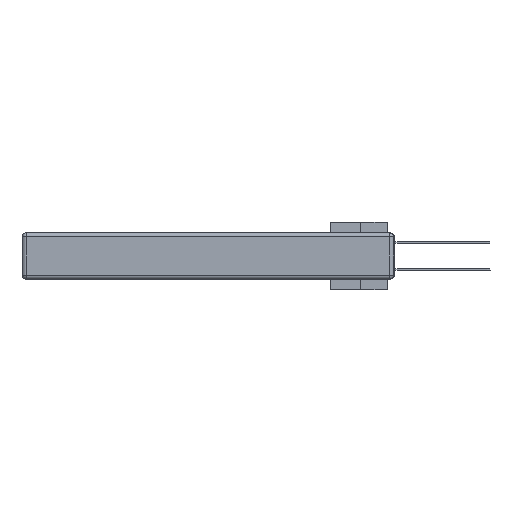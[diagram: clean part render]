
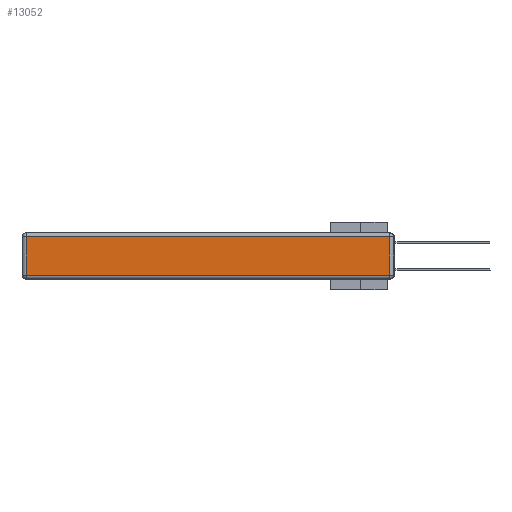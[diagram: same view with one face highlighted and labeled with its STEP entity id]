
A CAD part, left-side view. The second image highlights one B-rep face of the part: STEP entity #13052.
In plain terms, the highlighted planar face has unit normal (-1, 0, 0).
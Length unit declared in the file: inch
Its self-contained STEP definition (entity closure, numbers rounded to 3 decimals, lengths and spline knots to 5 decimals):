
#745 = ORIENTED_EDGE ( 'NONE', *, *, #20664, .T. ) ;
#1275 = DIRECTION ( 'NONE',  ( 0., 0., 1. ) ) ;
#3796 = VERTEX_POINT ( 'NONE', #12516 ) ;
#4359 = LINE ( 'NONE', #39683, #7560 ) ;
#4590 = AXIS2_PLACEMENT_3D ( 'NONE', #29711, #14274, #1275 ) ;
#4713 = PLANE ( 'NONE',  #4590 ) ;
#5811 = ORIENTED_EDGE ( 'NONE', *, *, #21199, .T. ) ;
#6497 = CARTESIAN_POINT ( 'NONE',  ( 0., 2.72, -0.03 ) ) ;
#7235 = VECTOR ( 'NONE', #10796, 39.37008 ) ;
#7301 = ORIENTED_EDGE ( 'NONE', *, *, #15232, .T. ) ;
#7560 = VECTOR ( 'NONE', #21020, 39.37008 ) ;
#10796 = DIRECTION ( 'NONE',  ( 0., 1., 0. ) ) ;
#12516 = CARTESIAN_POINT ( 'NONE',  ( 0., 0.03, -0.03 ) ) ;
#12968 = VERTEX_POINT ( 'NONE', #16524 ) ;
#13052 = ADVANCED_FACE ( 'NONE', ( #35187 ), #4713, .T. ) ;
#13236 = ORIENTED_EDGE ( 'NONE', *, *, #34912, .T. ) ;
#14274 = DIRECTION ( 'NONE',  ( -1., 0., 0. ) ) ;
#15232 = EDGE_CURVE ( 'NONE', #38771, #3796, #17478, .T. ) ;
#16524 = CARTESIAN_POINT ( 'NONE',  ( 0., 2.72, -0.313 ) ) ;
#17478 = LINE ( 'NONE', #39194, #26094 ) ;
#19481 = VERTEX_POINT ( 'NONE', #6497 ) ;
#20664 = EDGE_CURVE ( 'NONE', #12968, #38771, #4359, .T. ) ;
#21020 = DIRECTION ( 'NONE',  ( 0., -1., 0. ) ) ;
#21121 = DIRECTION ( 'NONE',  ( 0., 0., 1. ) ) ;
#21199 = EDGE_CURVE ( 'NONE', #19481, #12968, #36755, .T. ) ;
#24370 = CARTESIAN_POINT ( 'NONE',  ( 0., 0.03, -0.313 ) ) ;
#24452 = VECTOR ( 'NONE', #39593, 39.37008 ) ;
#26094 = VECTOR ( 'NONE', #21121, 39.37008 ) ;
#27986 = CARTESIAN_POINT ( 'NONE',  ( 0., 2.72, -0.343 ) ) ;
#29711 = CARTESIAN_POINT ( 'NONE',  ( 0., 0., -0.343 ) ) ;
#32322 = LINE ( 'NONE', #38404, #7235 ) ;
#32514 = EDGE_LOOP ( 'NONE', ( #745, #7301, #13236, #5811 ) ) ;
#34912 = EDGE_CURVE ( 'NONE', #3796, #19481, #32322, .T. ) ;
#35187 = FACE_OUTER_BOUND ( 'NONE', #32514, .T. ) ;
#36755 = LINE ( 'NONE', #27986, #24452 ) ;
#38404 = CARTESIAN_POINT ( 'NONE',  ( 0., 2.75, -0.03 ) ) ;
#38771 = VERTEX_POINT ( 'NONE', #24370 ) ;
#39194 = CARTESIAN_POINT ( 'NONE',  ( 0., 0.03, -0.343 ) ) ;
#39593 = DIRECTION ( 'NONE',  ( 0., 0., -1. ) ) ;
#39683 = CARTESIAN_POINT ( 'NONE',  ( 0., 0., -0.313 ) ) ;
